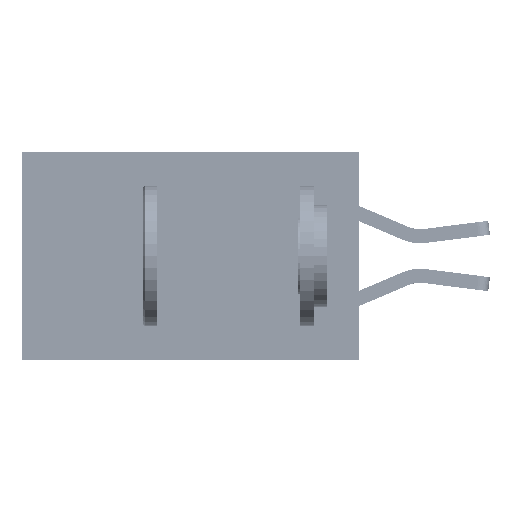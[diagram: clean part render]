
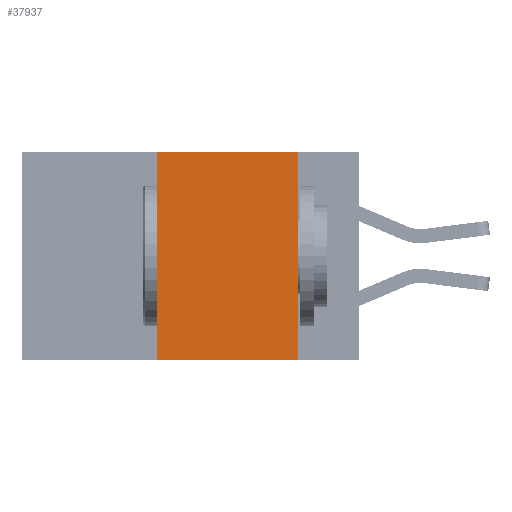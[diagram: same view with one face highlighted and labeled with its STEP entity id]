
A CAD part, left-side view. The second image highlights one B-rep face of the part: STEP entity #37937.
In plain terms, the highlighted planar face has unit normal (-1, 0, 0).
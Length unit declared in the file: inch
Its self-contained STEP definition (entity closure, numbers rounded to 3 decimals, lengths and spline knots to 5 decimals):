
#867 = CARTESIAN_POINT ( 'NONE',  ( 0., 0.11, 0. ) ) ;
#949 = EDGE_CURVE ( 'NONE', #19787, #35269, #22587, .T. ) ;
#1151 = CARTESIAN_POINT ( 'NONE',  ( 0., 0.36, 0. ) ) ;
#1485 = CARTESIAN_POINT ( 'NONE',  ( 0., 0.36, 0. ) ) ;
#3520 = VECTOR ( 'NONE', #21999, 39.37008 ) ;
#3634 = AXIS2_PLACEMENT_3D ( 'NONE', #36617, #19729, #43454 ) ;
#9036 = CARTESIAN_POINT ( 'NONE',  ( 0., 0.11, 0. ) ) ;
#9184 = CARTESIAN_POINT ( 'NONE',  ( 0., 0.36, -0.37 ) ) ;
#10390 = ORIENTED_EDGE ( 'NONE', *, *, #949, .F. ) ;
#12012 = LINE ( 'NONE', #14740, #30143 ) ;
#12852 = LINE ( 'NONE', #1151, #3520 ) ;
#13668 = ORIENTED_EDGE ( 'NONE', *, *, #34166, .T. ) ;
#14604 = DIRECTION ( 'NONE',  ( 0., -1., 0. ) ) ;
#14740 = CARTESIAN_POINT ( 'NONE',  ( 0., 0.6, -0.37 ) ) ;
#16290 = PLANE ( 'NONE',  #3634 ) ;
#16809 = EDGE_CURVE ( 'NONE', #19834, #18765, #12852, .T. ) ;
#18765 = VERTEX_POINT ( 'NONE', #1485 ) ;
#19011 = CARTESIAN_POINT ( 'NONE',  ( 0., 0.11, -0.37 ) ) ;
#19729 = DIRECTION ( 'NONE',  ( 1., 0., 0. ) ) ;
#19761 = FACE_OUTER_BOUND ( 'NONE', #43935, .T. ) ;
#19787 = VERTEX_POINT ( 'NONE', #9036 ) ;
#19834 = VERTEX_POINT ( 'NONE', #9184 ) ;
#21999 = DIRECTION ( 'NONE',  ( 0., 0., 1. ) ) ;
#22587 = LINE ( 'NONE', #867, #29459 ) ;
#23938 = DIRECTION ( 'NONE',  ( 0., -1., 0. ) ) ;
#25146 = DIRECTION ( 'NONE',  ( 0., 0., -1. ) ) ;
#25744 = EDGE_CURVE ( 'NONE', #18765, #19787, #26184, .T. ) ;
#26184 = LINE ( 'NONE', #27177, #43140 ) ;
#27177 = CARTESIAN_POINT ( 'NONE',  ( 0., 0.6, 0. ) ) ;
#29459 = VECTOR ( 'NONE', #25146, 39.37008 ) ;
#30143 = VECTOR ( 'NONE', #14604, 39.37008 ) ;
#34166 = EDGE_CURVE ( 'NONE', #19834, #35269, #12012, .T. ) ;
#35269 = VERTEX_POINT ( 'NONE', #19011 ) ;
#36617 = CARTESIAN_POINT ( 'NONE',  ( 0., 0.6, 0. ) ) ;
#37571 = ORIENTED_EDGE ( 'NONE', *, *, #25744, .F. ) ;
#37937 = ADVANCED_FACE ( 'NONE', ( #19761 ), #16290, .F. ) ;
#39683 = ORIENTED_EDGE ( 'NONE', *, *, #16809, .F. ) ;
#43140 = VECTOR ( 'NONE', #23938, 39.37008 ) ;
#43454 = DIRECTION ( 'NONE',  ( 0., 0., -1. ) ) ;
#43935 = EDGE_LOOP ( 'NONE', ( #10390, #37571, #39683, #13668 ) ) ;
